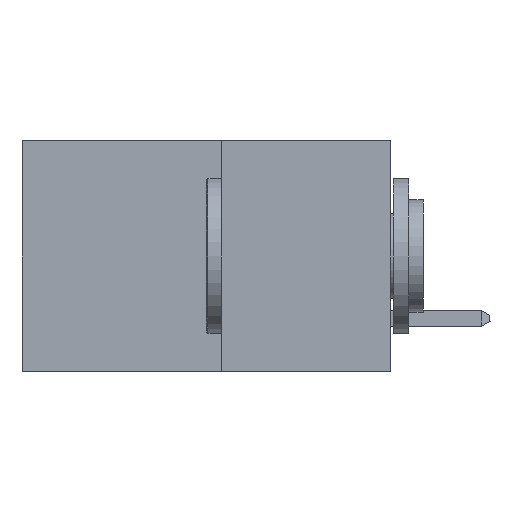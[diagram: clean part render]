
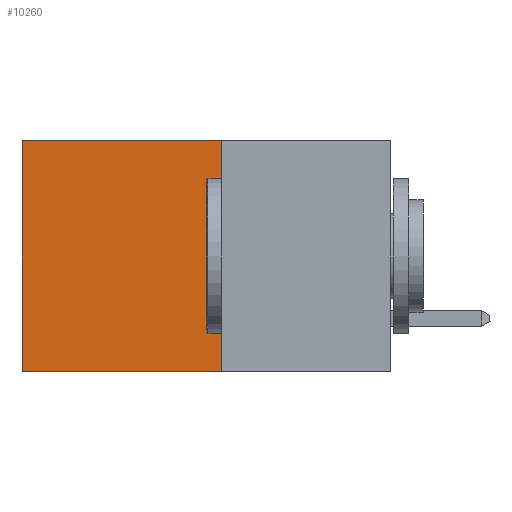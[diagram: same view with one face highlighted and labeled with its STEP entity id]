
A CAD part, left-side view. The second image highlights one B-rep face of the part: STEP entity #10260.
In plain terms, the highlighted planar face has unit normal (-1, 0, 0).
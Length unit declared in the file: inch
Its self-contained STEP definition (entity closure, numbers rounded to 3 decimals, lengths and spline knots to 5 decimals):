
#385 = CARTESIAN_POINT ( 'NONE',  ( 0.277, 0.27, 0. ) ) ;
#755 = ORIENTED_EDGE ( 'NONE', *, *, #23488, .T. ) ;
#1380 = CARTESIAN_POINT ( 'NONE',  ( 0.277, 0.59, -0.37 ) ) ;
#1474 = DIRECTION ( 'NONE',  ( 0., 0., -1. ) ) ;
#1799 = EDGE_CURVE ( 'NONE', #14131, #11933, #19447, .T. ) ;
#1802 = VECTOR ( 'NONE', #17666, 39.37008 ) ;
#1923 = ORIENTED_EDGE ( 'NONE', *, *, #1799, .F. ) ;
#2059 = LINE ( 'NONE', #20262, #7029 ) ;
#3318 = DIRECTION ( 'NONE',  ( 0., 0., -1. ) ) ;
#4702 = VECTOR ( 'NONE', #6343, 39.37008 ) ;
#5131 = CARTESIAN_POINT ( 'NONE',  ( 0.277, 0.27, -0.37 ) ) ;
#6121 = EDGE_CURVE ( 'NONE', #14131, #7157, #21444, .T. ) ;
#6343 = DIRECTION ( 'NONE',  ( 0., 0., -1. ) ) ;
#6785 = EDGE_CURVE ( 'NONE', #11933, #21353, #2059, .T. ) ;
#6869 = LINE ( 'NONE', #14506, #7451 ) ;
#7029 = VECTOR ( 'NONE', #20337, 39.37008 ) ;
#7082 = CARTESIAN_POINT ( 'NONE',  ( 0.277, 0.27, -0.37 ) ) ;
#7157 = VERTEX_POINT ( 'NONE', #14310 ) ;
#7451 = VECTOR ( 'NONE', #3318, 39.37008 ) ;
#10031 = AXIS2_PLACEMENT_3D ( 'NONE', #5131, #12630, #1474 ) ;
#10260 = ADVANCED_FACE ( 'NONE', ( #21839 ), #23528, .F. ) ;
#11933 = VERTEX_POINT ( 'NONE', #16721 ) ;
#12630 = DIRECTION ( 'NONE',  ( 1., 0., 0. ) ) ;
#13693 = ORIENTED_EDGE ( 'NONE', *, *, #6785, .F. ) ;
#14131 = VERTEX_POINT ( 'NONE', #385 ) ;
#14310 = CARTESIAN_POINT ( 'NONE',  ( 0.277, 0.59, 0. ) ) ;
#14506 = CARTESIAN_POINT ( 'NONE',  ( 0.277, 0.59, -0.37 ) ) ;
#15800 = EDGE_LOOP ( 'NONE', ( #755, #13693, #1923, #19253 ) ) ;
#16721 = CARTESIAN_POINT ( 'NONE',  ( 0.277, 0.27, -0.37 ) ) ;
#17666 = DIRECTION ( 'NONE',  ( 0., 1., 0. ) ) ;
#17760 = CARTESIAN_POINT ( 'NONE',  ( 0.277, 0.27, 0. ) ) ;
#19253 = ORIENTED_EDGE ( 'NONE', *, *, #6121, .T. ) ;
#19447 = LINE ( 'NONE', #7082, #4702 ) ;
#20262 = CARTESIAN_POINT ( 'NONE',  ( 0.277, 0.27, -0.37 ) ) ;
#20337 = DIRECTION ( 'NONE',  ( 0., 1., 0. ) ) ;
#21353 = VERTEX_POINT ( 'NONE', #1380 ) ;
#21444 = LINE ( 'NONE', #17760, #1802 ) ;
#21839 = FACE_OUTER_BOUND ( 'NONE', #15800, .T. ) ;
#23488 = EDGE_CURVE ( 'NONE', #7157, #21353, #6869, .T. ) ;
#23528 = PLANE ( 'NONE',  #10031 ) ;
